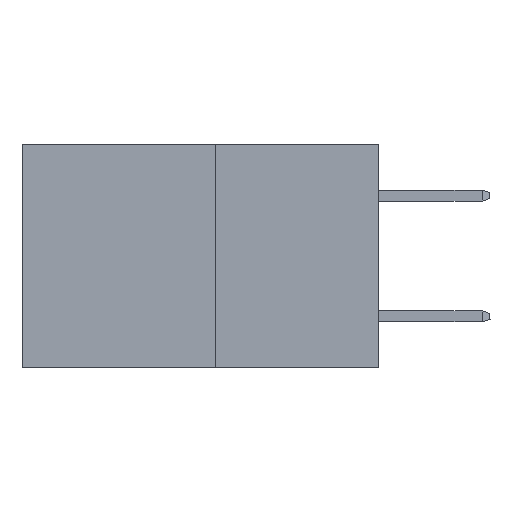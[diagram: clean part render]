
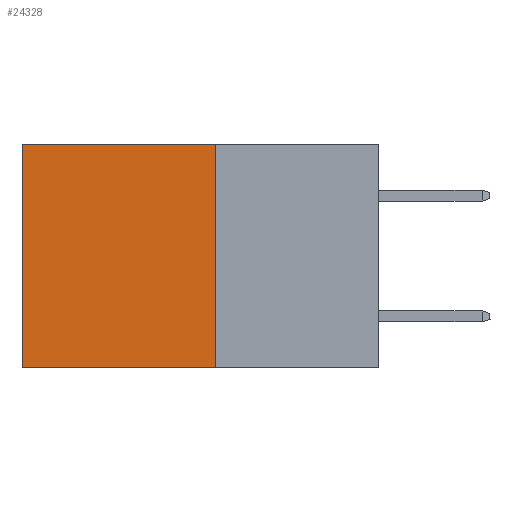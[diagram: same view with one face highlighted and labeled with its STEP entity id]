
A CAD part, left-side view. The second image highlights one B-rep face of the part: STEP entity #24328.
In plain terms, the highlighted planar face has unit normal (-1, 0, 0).
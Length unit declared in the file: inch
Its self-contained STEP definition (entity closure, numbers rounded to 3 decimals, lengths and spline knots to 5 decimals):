
#2375 = ORIENTED_EDGE ( 'NONE', *, *, #11692, .F. ) ;
#3138 = EDGE_LOOP ( 'NONE', ( #24883, #2375, #4569, #7117 ) ) ;
#4037 = VERTEX_POINT ( 'NONE', #28925 ) ;
#4569 = ORIENTED_EDGE ( 'NONE', *, *, #7562, .F. ) ;
#5185 = LINE ( 'NONE', #30503, #25712 ) ;
#6877 = CARTESIAN_POINT ( 'NONE',  ( 0.277, 0.27, -0.37 ) ) ;
#7082 = DIRECTION ( 'NONE',  ( 0., 0., -1. ) ) ;
#7117 = ORIENTED_EDGE ( 'NONE', *, *, #32824, .T. ) ;
#7562 = EDGE_CURVE ( 'NONE', #32591, #4037, #18234, .T. ) ;
#8742 = VERTEX_POINT ( 'NONE', #22465 ) ;
#9129 = VECTOR ( 'NONE', #21479, 39.37008 ) ;
#11109 = VECTOR ( 'NONE', #7082, 39.37008 ) ;
#11336 = AXIS2_PLACEMENT_3D ( 'NONE', #30523, #14487, #33221 ) ;
#11692 = EDGE_CURVE ( 'NONE', #4037, #8742, #21549, .T. ) ;
#11777 = DIRECTION ( 'NONE',  ( 0., 0., -1. ) ) ;
#14487 = DIRECTION ( 'NONE',  ( 1., 0., 0. ) ) ;
#14785 = CARTESIAN_POINT ( 'NONE',  ( 0.277, 0.59, 0. ) ) ;
#18234 = LINE ( 'NONE', #25665, #11109 ) ;
#21479 = DIRECTION ( 'NONE',  ( 0., 1., 0. ) ) ;
#21549 = LINE ( 'NONE', #6877, #27825 ) ;
#22442 = PLANE ( 'NONE',  #11336 ) ;
#22465 = CARTESIAN_POINT ( 'NONE',  ( 0.277, 0.59, -0.37 ) ) ;
#23372 = LINE ( 'NONE', #24307, #9129 ) ;
#23436 = CARTESIAN_POINT ( 'NONE',  ( 0.277, 0.27, 0. ) ) ;
#24307 = CARTESIAN_POINT ( 'NONE',  ( 0.277, 0.27, 0. ) ) ;
#24328 = ADVANCED_FACE ( 'NONE', ( #34740 ), #22442, .F. ) ;
#24883 = ORIENTED_EDGE ( 'NONE', *, *, #28826, .T. ) ;
#25665 = CARTESIAN_POINT ( 'NONE',  ( 0.277, 0.27, -0.37 ) ) ;
#25712 = VECTOR ( 'NONE', #11777, 39.37008 ) ;
#27825 = VECTOR ( 'NONE', #28403, 39.37008 ) ;
#28403 = DIRECTION ( 'NONE',  ( 0., 1., 0. ) ) ;
#28826 = EDGE_CURVE ( 'NONE', #29639, #8742, #5185, .T. ) ;
#28925 = CARTESIAN_POINT ( 'NONE',  ( 0.277, 0.27, -0.37 ) ) ;
#29639 = VERTEX_POINT ( 'NONE', #14785 ) ;
#30503 = CARTESIAN_POINT ( 'NONE',  ( 0.277, 0.59, -0.37 ) ) ;
#30523 = CARTESIAN_POINT ( 'NONE',  ( 0.277, 0.27, -0.37 ) ) ;
#32591 = VERTEX_POINT ( 'NONE', #23436 ) ;
#32824 = EDGE_CURVE ( 'NONE', #32591, #29639, #23372, .T. ) ;
#33221 = DIRECTION ( 'NONE',  ( 0., 0., -1. ) ) ;
#34740 = FACE_OUTER_BOUND ( 'NONE', #3138, .T. ) ;
